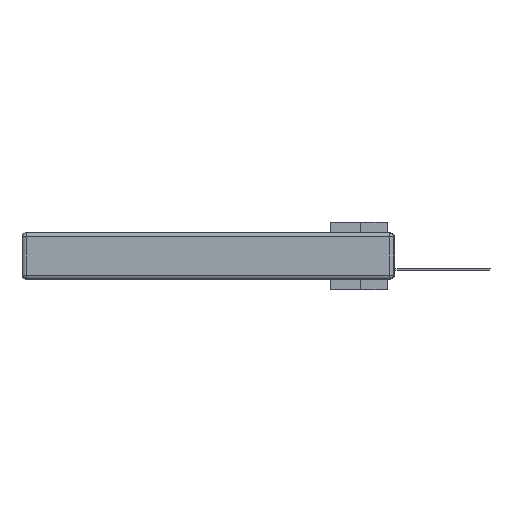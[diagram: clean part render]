
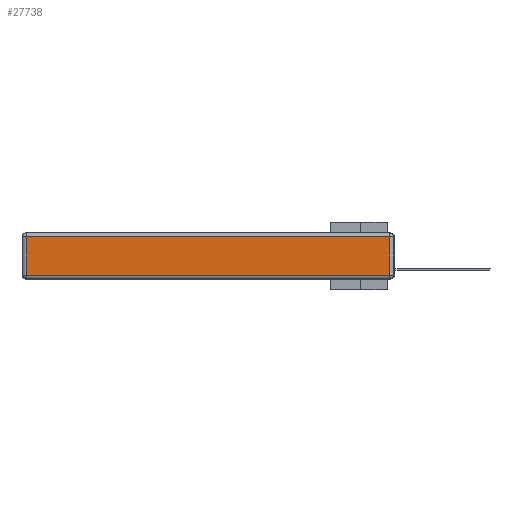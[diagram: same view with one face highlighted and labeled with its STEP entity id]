
A CAD part, left-side view. The second image highlights one B-rep face of the part: STEP entity #27738.
In plain terms, the highlighted planar face has unit normal (-1, 0, 0).
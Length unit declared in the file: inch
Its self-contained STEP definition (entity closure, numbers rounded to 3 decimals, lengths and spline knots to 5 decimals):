
#153 = EDGE_CURVE ( 'NONE', #10212, #23188, #14228, .T. ) ;
#171 = ORIENTED_EDGE ( 'NONE', *, *, #24368, .T. ) ;
#693 = LINE ( 'NONE', #32724, #7272 ) ;
#3207 = AXIS2_PLACEMENT_3D ( 'NONE', #5713, #33455, #11276 ) ;
#5145 = CARTESIAN_POINT ( 'NONE',  ( 0., 2.72, -0.03 ) ) ;
#5713 = CARTESIAN_POINT ( 'NONE',  ( 0., 0., -0.343 ) ) ;
#6167 = CARTESIAN_POINT ( 'NONE',  ( 0., 0.03, -0.313 ) ) ;
#6876 = VECTOR ( 'NONE', #26076, 39.37008 ) ;
#7074 = VERTEX_POINT ( 'NONE', #6167 ) ;
#7272 = VECTOR ( 'NONE', #21144, 39.37008 ) ;
#7274 = CARTESIAN_POINT ( 'NONE',  ( 0., 2.72, -0.343 ) ) ;
#8236 = EDGE_CURVE ( 'NONE', #23188, #30440, #18836, .T. ) ;
#9902 = CARTESIAN_POINT ( 'NONE',  ( 0., 0.03, -0.03 ) ) ;
#10039 = CARTESIAN_POINT ( 'NONE',  ( 0., 2.75, -0.03 ) ) ;
#10212 = VERTEX_POINT ( 'NONE', #9902 ) ;
#11276 = DIRECTION ( 'NONE',  ( 0., 0., 1. ) ) ;
#12689 = DIRECTION ( 'NONE',  ( 0., -1., 0. ) ) ;
#14228 = LINE ( 'NONE', #10039, #6876 ) ;
#15908 = CARTESIAN_POINT ( 'NONE',  ( 0., 2.72, -0.313 ) ) ;
#16389 = ORIENTED_EDGE ( 'NONE', *, *, #8236, .T. ) ;
#18836 = LINE ( 'NONE', #7274, #21870 ) ;
#21101 = VECTOR ( 'NONE', #12689, 39.37008 ) ;
#21144 = DIRECTION ( 'NONE',  ( 0., 0., 1. ) ) ;
#21856 = EDGE_LOOP ( 'NONE', ( #28557, #171, #34149, #16389 ) ) ;
#21870 = VECTOR ( 'NONE', #29701, 39.37008 ) ;
#22391 = LINE ( 'NONE', #29218, #21101 ) ;
#23188 = VERTEX_POINT ( 'NONE', #5145 ) ;
#24112 = EDGE_CURVE ( 'NONE', #30440, #7074, #22391, .T. ) ;
#24368 = EDGE_CURVE ( 'NONE', #7074, #10212, #693, .T. ) ;
#24942 = FACE_OUTER_BOUND ( 'NONE', #21856, .T. ) ;
#26076 = DIRECTION ( 'NONE',  ( 0., 1., 0. ) ) ;
#27738 = ADVANCED_FACE ( 'NONE', ( #24942 ), #30803, .T. ) ;
#28557 = ORIENTED_EDGE ( 'NONE', *, *, #24112, .T. ) ;
#29218 = CARTESIAN_POINT ( 'NONE',  ( 0., 0., -0.313 ) ) ;
#29701 = DIRECTION ( 'NONE',  ( 0., 0., -1. ) ) ;
#30440 = VERTEX_POINT ( 'NONE', #15908 ) ;
#30803 = PLANE ( 'NONE',  #3207 ) ;
#32724 = CARTESIAN_POINT ( 'NONE',  ( 0., 0.03, -0.343 ) ) ;
#33455 = DIRECTION ( 'NONE',  ( -1., 0., 0. ) ) ;
#34149 = ORIENTED_EDGE ( 'NONE', *, *, #153, .T. ) ;
